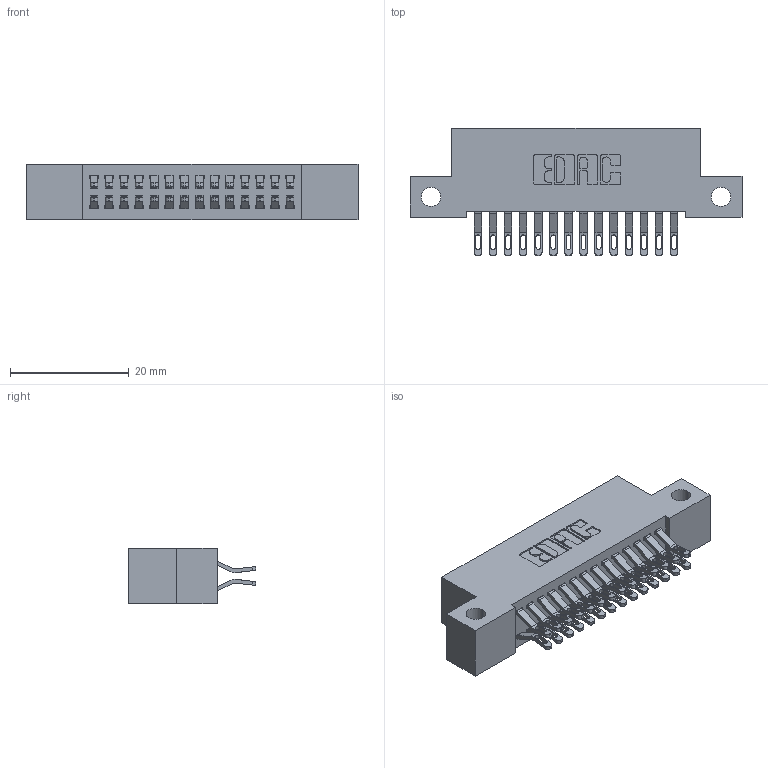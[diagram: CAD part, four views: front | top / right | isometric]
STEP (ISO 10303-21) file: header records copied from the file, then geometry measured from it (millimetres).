
FILE_DESCRIPTION (( 'STEP AP203' ), '1' );
FILE_NAME ('342-028-555-212.STEP', '2018-08-11T14:26:10', ( '' ), ( '' ), 'SwSTEP 2.0', 'SolidWorks 2016', '' );
FILE_SCHEMA (( 'CONFIG_CONTROL_DESIGN' ));
Length unit declared in the file: inch
Products named in the file (3): 342 Part_Side Mount; 345-292-001_555 Tail; 342-028-555-212
Assembly tree (29 placements, depth 2):
  342-028-555-212
    342 Part_Side Mount
    345-292-001_555 Tail  x28
Bounding box: 55.88 x 21.47 x 9.4 mm (x, y, z)
Volume: 4892.2 mm3; surface area: 7384.4 mm2
Topology: 29 solids, 29 shells, 1734 faces, 5423 edges, 3614 vertices
Faces by surface type: plane 1018, cylinder 716
Entity records: 12825 total; most frequent: CARTESIAN_POINT 2192, ORIENTED_EDGE 2098, DIRECTION 1893, EDGE_CURVE 1049, VECTOR 901, LINE 901, VERTEX_POINT 698, AXIS2_PLACEMENT_3D 496
